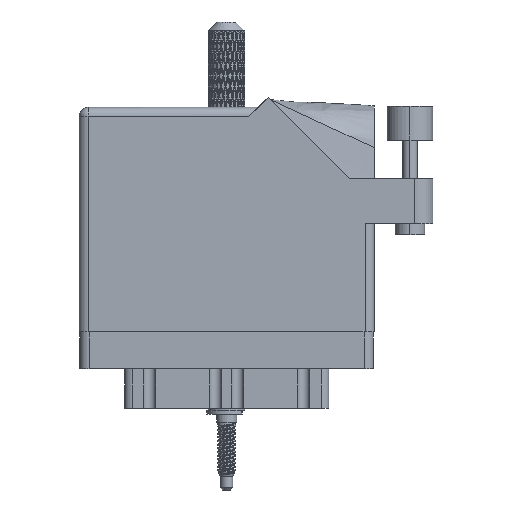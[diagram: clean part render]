
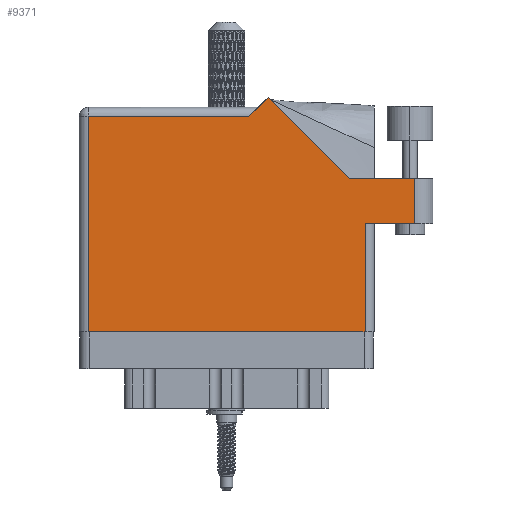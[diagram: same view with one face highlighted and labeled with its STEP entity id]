
A CAD part, front view. The second image highlights one B-rep face of the part: STEP entity #9371.
In plain terms, the highlighted face is planar.
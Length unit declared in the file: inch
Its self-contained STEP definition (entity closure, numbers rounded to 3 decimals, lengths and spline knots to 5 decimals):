
#1042 = VECTOR ( 'NONE', #73079, 39.37008 ) ;
#3490 = LINE ( 'NONE', #67513, #27295 ) ;
#5825 = CARTESIAN_POINT ( 'NONE',  ( 1.948, 0., 0. ) ) ;
#6480 = CARTESIAN_POINT ( 'NONE',  ( 0.062, 0., 0. ) ) ;
#6622 = CARTESIAN_POINT ( 'NONE',  ( 2.285, 1.044, 0. ) ) ;
#6862 = DIRECTION ( 'NONE',  ( -1., 0., 0. ) ) ;
#9371 = ADVANCED_FACE ( 'NONE', ( #31648 ), #72358, .F. ) ;
#11552 = EDGE_LOOP ( 'NONE', ( #76004, #66658, #51597, #42029, #37692, #19435, #97995, #19993, #73335 ) ) ;
#11888 = EDGE_CURVE ( 'NONE', #104228, #74440, #87656, .T. ) ;
#14027 = DIRECTION ( 'NONE',  ( 1., 0., 0. ) ) ;
#14303 = LINE ( 'NONE', #21713, #95564 ) ;
#14502 = LINE ( 'NONE', #72625, #50680 ) ;
#15079 = CARTESIAN_POINT ( 'NONE',  ( 2.01, 0.737, 0. ) ) ;
#19435 = ORIENTED_EDGE ( 'NONE', *, *, #79142, .T. ) ;
#19993 = ORIENTED_EDGE ( 'NONE', *, *, #89953, .T. ) ;
#21713 = CARTESIAN_POINT ( 'NONE',  ( 0., 1.468, 0. ) ) ;
#23553 = LINE ( 'NONE', #15079, #45666 ) ;
#24122 = LINE ( 'NONE', #6622, #75604 ) ;
#25600 = CARTESIAN_POINT ( 'NONE',  ( 1.84442, 1.044, 0. ) ) ;
#26163 = CARTESIAN_POINT ( 'NONE',  ( 1.217, 1.53, 0. ) ) ;
#27295 = VECTOR ( 'NONE', #68560, 39.37008 ) ;
#31648 = FACE_OUTER_BOUND ( 'NONE', #11552, .T. ) ;
#33737 = CARTESIAN_POINT ( 'NONE',  ( 1.948, 0.737, 0. ) ) ;
#37692 = ORIENTED_EDGE ( 'NONE', *, *, #93468, .T. ) ;
#39937 = DIRECTION ( 'NONE',  ( 0., 1., 0. ) ) ;
#40817 = CARTESIAN_POINT ( 'NONE',  ( 2.41, 1.044, 0. ) ) ;
#42029 = ORIENTED_EDGE ( 'NONE', *, *, #55777, .T. ) ;
#45666 = VECTOR ( 'NONE', #14027, 39.37008 ) ;
#48638 = VERTEX_POINT ( 'NONE', #85137 ) ;
#48848 = VERTEX_POINT ( 'NONE', #5825 ) ;
#50367 = CARTESIAN_POINT ( 'NONE',  ( 2.285, 1.044, 0. ) ) ;
#50680 = VECTOR ( 'NONE', #71597, 39.37008 ) ;
#50702 = LINE ( 'NONE', #52269, #77809 ) ;
#51242 = DIRECTION ( 'NONE',  ( 0., 1., 0. ) ) ;
#51573 = EDGE_CURVE ( 'NONE', #70317, #48638, #23553, .T. ) ;
#51597 = ORIENTED_EDGE ( 'NONE', *, *, #79044, .T. ) ;
#52269 = CARTESIAN_POINT ( 'NONE',  ( 1.948, 0.737, 0. ) ) ;
#55777 = EDGE_CURVE ( 'NONE', #57721, #90948, #14502, .T. ) ;
#57721 = VERTEX_POINT ( 'NONE', #25600 ) ;
#58437 = DIRECTION ( 'NONE',  ( -0.707, -0.707, 0. ) ) ;
#58464 = CARTESIAN_POINT ( 'NONE',  ( 0., 1.53, 0. ) ) ;
#58626 = EDGE_CURVE ( 'NONE', #48848, #70317, #50702, .T. ) ;
#58971 = DIRECTION ( 'NONE',  ( -1., 0., 0. ) ) ;
#65644 = VECTOR ( 'NONE', #103539, 39.37008 ) ;
#65828 = LINE ( 'NONE', #26163, #88297 ) ;
#66658 = ORIENTED_EDGE ( 'NONE', *, *, #83379, .T. ) ;
#67513 = CARTESIAN_POINT ( 'NONE',  ( 0., 0., 0. ) ) ;
#68560 = DIRECTION ( 'NONE',  ( 1., 0., 0. ) ) ;
#69229 = VERTEX_POINT ( 'NONE', #50367 ) ;
#70317 = VERTEX_POINT ( 'NONE', #33737 ) ;
#71597 = DIRECTION ( 'NONE',  ( -0.707, 0.707, 0. ) ) ;
#72358 = PLANE ( 'NONE',  #74057 ) ;
#72625 = CARTESIAN_POINT ( 'NONE',  ( 1.84442, 1.044, 0. ) ) ;
#73079 = DIRECTION ( 'NONE',  ( -1., 0., 0. ) ) ;
#73335 = ORIENTED_EDGE ( 'NONE', *, *, #58626, .T. ) ;
#74057 = AXIS2_PLACEMENT_3D ( 'NONE', #58464, #74262, #58971 ) ;
#74262 = DIRECTION ( 'NONE',  ( 0., 0., -1. ) ) ;
#74440 = VERTEX_POINT ( 'NONE', #6480 ) ;
#75604 = VECTOR ( 'NONE', #39937, 39.37008 ) ;
#76004 = ORIENTED_EDGE ( 'NONE', *, *, #51573, .T. ) ;
#76342 = CARTESIAN_POINT ( 'NONE',  ( 1.28771, 1.60071, 0. ) ) ;
#77809 = VECTOR ( 'NONE', #51242, 39.37008 ) ;
#79044 = EDGE_CURVE ( 'NONE', #69229, #57721, #88880, .T. ) ;
#79142 = EDGE_CURVE ( 'NONE', #92327, #104228, #14303, .T. ) ;
#83379 = EDGE_CURVE ( 'NONE', #48638, #69229, #24122, .T. ) ;
#85137 = CARTESIAN_POINT ( 'NONE',  ( 2.285, 0.737, 0. ) ) ;
#87656 = LINE ( 'NONE', #103007, #65644 ) ;
#88297 = VECTOR ( 'NONE', #58437, 39.37008 ) ;
#88880 = LINE ( 'NONE', #40817, #1042 ) ;
#89953 = EDGE_CURVE ( 'NONE', #74440, #48848, #3490, .T. ) ;
#90329 = CARTESIAN_POINT ( 'NONE',  ( 0.062, 1.468, 0. ) ) ;
#90948 = VERTEX_POINT ( 'NONE', #76342 ) ;
#92327 = VERTEX_POINT ( 'NONE', #97339 ) ;
#93468 = EDGE_CURVE ( 'NONE', #90948, #92327, #65828, .T. ) ;
#95564 = VECTOR ( 'NONE', #6862, 39.37008 ) ;
#97339 = CARTESIAN_POINT ( 'NONE',  ( 1.155, 1.468, 0. ) ) ;
#97995 = ORIENTED_EDGE ( 'NONE', *, *, #11888, .T. ) ;
#103007 = CARTESIAN_POINT ( 'NONE',  ( 0.062, 0., 0. ) ) ;
#103539 = DIRECTION ( 'NONE',  ( 0., -1., 0. ) ) ;
#104228 = VERTEX_POINT ( 'NONE', #90329 ) ;
